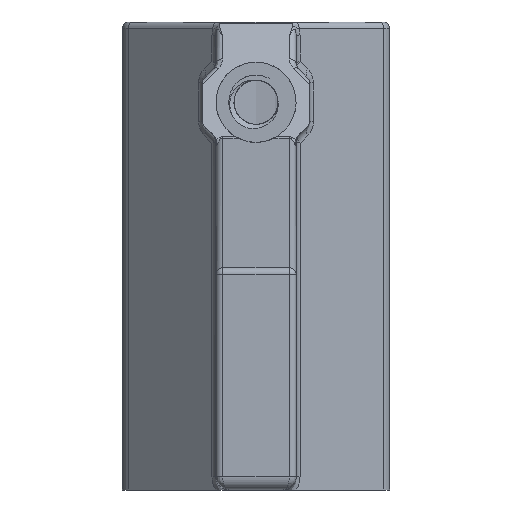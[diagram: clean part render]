
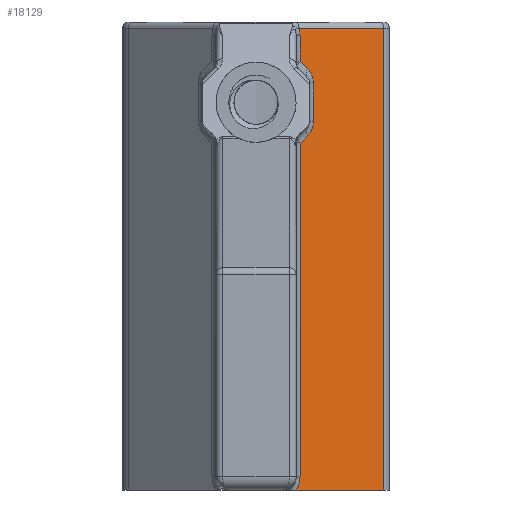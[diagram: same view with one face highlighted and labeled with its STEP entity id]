
A CAD part, front view. The second image highlights one B-rep face of the part: STEP entity #18129.
In plain terms, the highlighted planar face has unit normal (0.707, -0.707, 0).
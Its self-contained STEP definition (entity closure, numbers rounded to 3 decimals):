
#309 = VERTEX_POINT ( 'NONE', #25825 ) ;
#811 = CARTESIAN_POINT ( 'NONE',  ( 6.542, -28.458, 68.7 ) ) ;
#1030 = VERTEX_POINT ( 'NONE', #33465 ) ;
#2320 = LINE ( 'NONE', #8042, #24709 ) ;
#2507 = CARTESIAN_POINT ( 'NONE',  ( 8.586, -26.414, 55.101 ) ) ;
#2760 = EDGE_CURVE ( 'NONE', #5227, #26535, #22639, .T. ) ;
#2908 = EDGE_CURVE ( 'NONE', #43322, #16523, #36706, .T. ) ;
#3149 = CARTESIAN_POINT ( 'NONE',  ( 8.179, -26.821, 62.549 ) ) ;
#3828 = CARTESIAN_POINT ( 'NONE',  ( 8.277, -26.723, 53.549 ) ) ;
#5154 = CARTESIAN_POINT ( 'NONE',  ( 6.586, -28.414, 63.728 ) ) ;
#5227 = VERTEX_POINT ( 'NONE', #22016 ) ;
#5231 = ORIENTED_EDGE ( 'NONE', *, *, #11980, .T. ) ;
#5514 = CARTESIAN_POINT ( 'NONE',  ( 8.277, -26.723, 62.451 ) ) ;
#5867 = ORIENTED_EDGE ( 'NONE', *, *, #2908, .T. ) ;
#5884 = CARTESIAN_POINT ( 'NONE',  ( 20., -15., 70. ) ) ;
#6024 = EDGE_CURVE ( 'NONE', #17110, #1030, #21557, .T. ) ;
#7475 = LINE ( 'NONE', #12085, #45670 ) ;
#7605 = VECTOR ( 'NONE', #16364, 1000. ) ;
#7728 = CARTESIAN_POINT ( 'NONE',  ( 6.586, -28.414, 2. ) ) ;
#8042 = CARTESIAN_POINT ( 'NONE',  ( 20., -15., 0. ) ) ;
#9053 = EDGE_CURVE ( 'NONE', #50645, #17110, #2320, .T. ) ;
#9440 = CARTESIAN_POINT ( 'NONE',  ( 6.457, -28.543, 69. ) ) ;
#10032 = ORIENTED_EDGE ( 'NONE', *, *, #46223, .T. ) ;
#10577 = DIRECTION ( 'NONE',  ( 0., 0., -1. ) ) ;
#11888 = CARTESIAN_POINT ( 'NONE',  ( 7.707, -27.293, 52.979 ) ) ;
#11980 = EDGE_CURVE ( 'NONE', #32042, #24894, #24135, .T. ) ;
#12085 = CARTESIAN_POINT ( 'NONE',  ( 6., -29., 69. ) ) ;
#12334 = CARTESIAN_POINT ( 'NONE',  ( 6.05, -28.95, 0. ) ) ;
#12461 = CARTESIAN_POINT ( 'NONE',  ( 8.586, -26.414, 55.101 ) ) ;
#12468 = ORIENTED_EDGE ( 'NONE', *, *, #9053, .T. ) ;
#13220 = DIRECTION ( 'NONE',  ( 0., 0., -1. ) ) ;
#14496 = ORIENTED_EDGE ( 'NONE', *, *, #32172, .T. ) ;
#14597 = CARTESIAN_POINT ( 'NONE',  ( 6.586, -28.414, 67.96 ) ) ;
#14945 =( BOUNDED_CURVE ( )  B_SPLINE_CURVE ( 3, ( #12461, #52071, #3828, #11888 ),
 .UNSPECIFIED., .F., .F. ) 
 B_SPLINE_CURVE_WITH_KNOTS ( ( 4, 4 ),
 ( 0., 0.785 ),
 .UNSPECIFIED. ) 
 CURVE ( )  GEOMETRIC_REPRESENTATION_ITEM ( )  RATIONAL_B_SPLINE_CURVE ( ( 1., 0.949, 0.949, 1. ) ) 
 REPRESENTATION_ITEM ( '' )  );
#15574 = ORIENTED_EDGE ( 'NONE', *, *, #17350, .T. ) ;
#16364 = DIRECTION ( 'NONE',  ( 0.577, 0.577, -0.577 ) ) ;
#16523 = VERTEX_POINT ( 'NONE', #46133 ) ;
#17110 = VERTEX_POINT ( 'NONE', #47490 ) ;
#17124 =( BOUNDED_CURVE ( )  B_SPLINE_CURVE ( 3, ( #22753, #5514, #17876, #52913 ),
 .UNSPECIFIED., .F., .F. ) 
 B_SPLINE_CURVE_WITH_KNOTS ( ( 4, 4 ),
 ( 5.498, 6.283 ),
 .UNSPECIFIED. ) 
 CURVE ( )  GEOMETRIC_REPRESENTATION_ITEM ( )  RATIONAL_B_SPLINE_CURVE ( ( 1., 0.949, 0.949, 1. ) ) 
 REPRESENTATION_ITEM ( '' )  );
#17350 = EDGE_CURVE ( 'NONE', #24894, #43322, #17124, .T. ) ;
#17876 = CARTESIAN_POINT ( 'NONE',  ( 8.586, -26.414, 61.706 ) ) ;
#17926 = ORIENTED_EDGE ( 'NONE', *, *, #28864, .T. ) ;
#18129 = ADVANCED_FACE ( 'NONE', ( #26856 ), #44088, .F. ) ;
#18859 = ORIENTED_EDGE ( 'NONE', *, *, #53352, .T. ) ;
#21557 = LINE ( 'NONE', #21822, #40679 ) ;
#21822 = CARTESIAN_POINT ( 'NONE',  ( 19.121, -15.879, 70. ) ) ;
#21866 = EDGE_CURVE ( 'NONE', #27196, #50645, #33230, .T. ) ;
#22016 = CARTESIAN_POINT ( 'NONE',  ( 7.707, -27.293, 52.979 ) ) ;
#22639 = LINE ( 'NONE', #26661, #42427 ) ;
#22753 = CARTESIAN_POINT ( 'NONE',  ( 7.707, -27.293, 63.021 ) ) ;
#23868 = LINE ( 'NONE', #41684, #36532 ) ;
#24135 = LINE ( 'NONE', #3149, #7605 ) ;
#24516 = CARTESIAN_POINT ( 'NONE',  ( 6.586, -28.414, 64.142 ) ) ;
#24709 = VECTOR ( 'NONE', #54873, 1000. ) ;
#24894 = VERTEX_POINT ( 'NONE', #33800 ) ;
#24965 = CARTESIAN_POINT ( 'NONE',  ( 6.586, -28.414, 67.96 ) ) ;
#25531 = CARTESIAN_POINT ( 'NONE',  ( 6.586, -28.414, 1.294 ) ) ;
#25825 = CARTESIAN_POINT ( 'NONE',  ( 6.457, -28.543, 69. ) ) ;
#26535 = VERTEX_POINT ( 'NONE', #46707 ) ;
#26661 = CARTESIAN_POINT ( 'NONE',  ( 6.764, -28.236, 52.036 ) ) ;
#26856 = FACE_OUTER_BOUND ( 'NONE', #31468, .T. ) ;
#27196 = VERTEX_POINT ( 'NONE', #39722 ) ;
#28864 = EDGE_CURVE ( 'NONE', #31389, #32042, #44220, .T. ) ;
#29823 = ORIENTED_EDGE ( 'NONE', *, *, #21866, .T. ) ;
#30365 =( BOUNDED_CURVE ( )  B_SPLINE_CURVE ( 3, ( #9440, #811, #31826, #14597 ),
 .UNSPECIFIED., .F., .F. ) 
 B_SPLINE_CURVE_WITH_KNOTS ( ( 4, 4 ),
 ( 3.427, 3.721 ),
 .UNSPECIFIED. ) 
 CURVE ( )  GEOMETRIC_REPRESENTATION_ITEM ( )  RATIONAL_B_SPLINE_CURVE ( ( 1., 0.993, 0.993, 1. ) ) 
 REPRESENTATION_ITEM ( '' )  );
#31389 = VERTEX_POINT ( 'NONE', #24965 ) ;
#31468 = EDGE_LOOP ( 'NONE', ( #56033, #18859, #10032, #17926, #5231, #15574, #5867, #14496, #35987, #43377, #29823, #12468 ) ) ;
#31826 = CARTESIAN_POINT ( 'NONE',  ( 6.586, -28.414, 68.351 ) ) ;
#32042 = VERTEX_POINT ( 'NONE', #24516 ) ;
#32172 = EDGE_CURVE ( 'NONE', #16523, #5227, #14945, .T. ) ;
#33230 =( BOUNDED_CURVE ( )  B_SPLINE_CURVE ( 3, ( #7728, #25531, #42776, #12334 ),
 .UNSPECIFIED., .F., .F. ) 
 B_SPLINE_CURVE_WITH_KNOTS ( ( 4, 4 ),
 ( 0., 0.524 ),
 .UNSPECIFIED. ) 
 CURVE ( )  GEOMETRIC_REPRESENTATION_ITEM ( )  RATIONAL_B_SPLINE_CURVE ( ( 1., 0.977, 0.977, 1. ) ) 
 REPRESENTATION_ITEM ( '' )  );
#33465 = CARTESIAN_POINT ( 'NONE',  ( 19.121, -15.879, 69. ) ) ;
#33800 = CARTESIAN_POINT ( 'NONE',  ( 7.707, -27.293, 63.021 ) ) ;
#35987 = ORIENTED_EDGE ( 'NONE', *, *, #2760, .T. ) ;
#36532 = VECTOR ( 'NONE', #41101, 1000. ) ;
#36706 = LINE ( 'NONE', #2507, #41533 ) ;
#36728 = VECTOR ( 'NONE', #13220, 1000. ) ;
#37026 = CARTESIAN_POINT ( 'NONE',  ( 6.05, -28.95, 0. ) ) ;
#38480 = DIRECTION ( 'NONE',  ( -0.707, -0.707, 0. ) ) ;
#39062 = DIRECTION ( 'NONE',  ( 0., 0., 1. ) ) ;
#39722 = CARTESIAN_POINT ( 'NONE',  ( 6.586, -28.414, 2. ) ) ;
#40679 = VECTOR ( 'NONE', #39062, 1000. ) ;
#40937 = CARTESIAN_POINT ( 'NONE',  ( 8.586, -26.414, 60.899 ) ) ;
#41101 = DIRECTION ( 'NONE',  ( 0., 0., -1. ) ) ;
#41533 = VECTOR ( 'NONE', #10577, 1000. ) ;
#41684 = CARTESIAN_POINT ( 'NONE',  ( 6.586, -28.414, 2. ) ) ;
#42051 = AXIS2_PLACEMENT_3D ( 'NONE', #5884, #45228, #44375 ) ;
#42427 = VECTOR ( 'NONE', #48772, 1000. ) ;
#42776 = CARTESIAN_POINT ( 'NONE',  ( 6.403, -28.597, 0.612 ) ) ;
#43322 = VERTEX_POINT ( 'NONE', #40937 ) ;
#43377 = ORIENTED_EDGE ( 'NONE', *, *, #54285, .T. ) ;
#44088 = PLANE ( 'NONE',  #42051 ) ;
#44220 = LINE ( 'NONE', #5154, #36728 ) ;
#44375 = DIRECTION ( 'NONE',  ( -0.707, -0.707, 0. ) ) ;
#45228 = DIRECTION ( 'NONE',  ( -0.707, 0.707, 0. ) ) ;
#45670 = VECTOR ( 'NONE', #38480, 1000. ) ;
#46133 = CARTESIAN_POINT ( 'NONE',  ( 8.586, -26.414, 55.101 ) ) ;
#46223 = EDGE_CURVE ( 'NONE', #309, #31389, #30365, .T. ) ;
#46707 = CARTESIAN_POINT ( 'NONE',  ( 6.586, -28.414, 51.858 ) ) ;
#47490 = CARTESIAN_POINT ( 'NONE',  ( 19.121, -15.879, 0. ) ) ;
#48772 = DIRECTION ( 'NONE',  ( -0.577, -0.577, -0.577 ) ) ;
#50645 = VERTEX_POINT ( 'NONE', #37026 ) ;
#52071 = CARTESIAN_POINT ( 'NONE',  ( 8.586, -26.414, 54.294 ) ) ;
#52913 = CARTESIAN_POINT ( 'NONE',  ( 8.586, -26.414, 60.899 ) ) ;
#53352 = EDGE_CURVE ( 'NONE', #1030, #309, #7475, .T. ) ;
#54285 = EDGE_CURVE ( 'NONE', #26535, #27196, #23868, .T. ) ;
#54873 = DIRECTION ( 'NONE',  ( 0.707, 0.707, 0. ) ) ;
#56033 = ORIENTED_EDGE ( 'NONE', *, *, #6024, .T. ) ;
